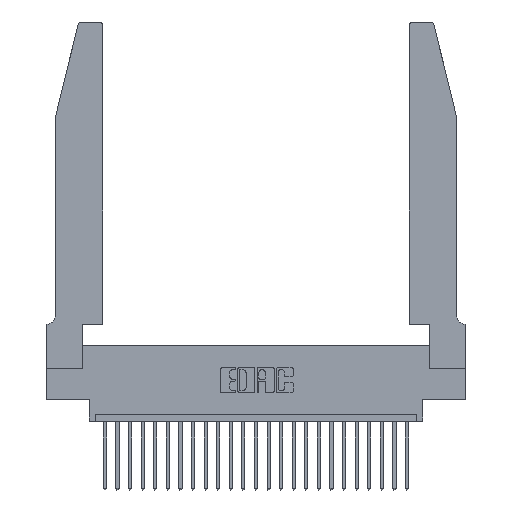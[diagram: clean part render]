
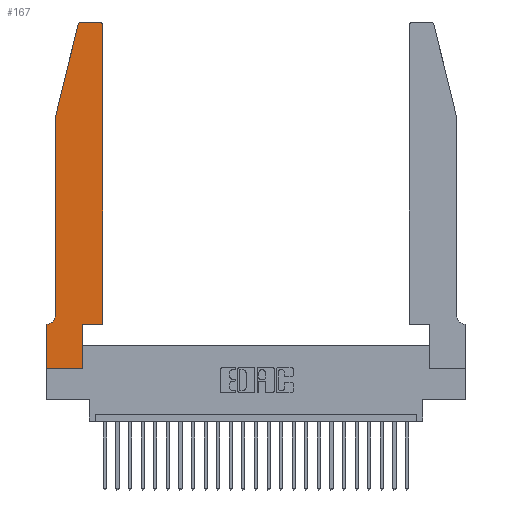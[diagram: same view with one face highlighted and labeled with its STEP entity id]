
A CAD part, top view. The second image highlights one B-rep face of the part: STEP entity #167.
In plain terms, the highlighted planar face has unit normal (0, 0, 1).
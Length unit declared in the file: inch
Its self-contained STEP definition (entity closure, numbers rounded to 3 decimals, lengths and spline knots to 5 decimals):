
#39 = DIRECTION ( 'NONE',  ( -1., 0., 0. ) ) ;
#167 = ADVANCED_FACE ( 'NONE', ( #18396 ), #13384, .T. ) ;
#365 = DIRECTION ( 'NONE',  ( 0., -1., 0. ) ) ;
#566 = VERTEX_POINT ( 'NONE', #7921 ) ;
#582 = CARTESIAN_POINT ( 'NONE',  ( 0.284, 2.72, 0.37 ) ) ;
#617 = VERTEX_POINT ( 'NONE', #24511 ) ;
#814 = EDGE_CURVE ( 'NONE', #566, #20338, #5829, .T. ) ;
#999 = VERTEX_POINT ( 'NONE', #2072 ) ;
#1170 = DIRECTION ( 'NONE',  ( 1., 0., 0. ) ) ;
#1643 = VECTOR ( 'NONE', #13195, 39.37008 ) ;
#1770 = ORIENTED_EDGE ( 'NONE', *, *, #11974, .T. ) ;
#1819 = LINE ( 'NONE', #13498, #22578 ) ;
#2072 = CARTESIAN_POINT ( 'NONE',  ( 0.4505, 0.35, 0.37 ) ) ;
#2327 = LINE ( 'NONE', #6353, #23367 ) ;
#2420 = EDGE_CURVE ( 'NONE', #9764, #12664, #5429, .T. ) ;
#2441 = LINE ( 'NONE', #2659, #17865 ) ;
#2659 = CARTESIAN_POINT ( 'NONE',  ( 0., 0., 0.37 ) ) ;
#3361 = ORIENTED_EDGE ( 'NONE', *, *, #10811, .T. ) ;
#4263 = DIRECTION ( 'NONE',  ( -1., 0., 0. ) ) ;
#4925 = EDGE_CURVE ( 'NONE', #22649, #25336, #2441, .T. ) ;
#5098 = CARTESIAN_POINT ( 'NONE',  ( 0.4505, 0.35, 0.37 ) ) ;
#5145 = LINE ( 'NONE', #5098, #1643 ) ;
#5199 = CARTESIAN_POINT ( 'NONE',  ( 0.0755, 2., 0.37 ) ) ;
#5429 = CIRCLE ( 'NONE', #22762, 0.07 ) ;
#5458 = AXIS2_PLACEMENT_3D ( 'NONE', #582, #18688, #22543 ) ;
#5829 = CIRCLE ( 'NONE', #11359, 0.03 ) ;
#5853 = LINE ( 'NONE', #8054, #14052 ) ;
#6013 = DIRECTION ( 'NONE',  ( 1., 0., 0. ) ) ;
#6155 = EDGE_LOOP ( 'NONE', ( #20588, #1770, #6347, #13376, #12126, #21054, #19779, #21338, #3361, #15868, #18955, #24180 ) ) ;
#6347 = ORIENTED_EDGE ( 'NONE', *, *, #15569, .T. ) ;
#6353 = CARTESIAN_POINT ( 'NONE',  ( 0.0755, 0.35, 0.37 ) ) ;
#6870 = EDGE_CURVE ( 'NONE', #25336, #15212, #14333, .T. ) ;
#6914 = CARTESIAN_POINT ( 'NONE',  ( 0.0055, 0.42, 0.37 ) ) ;
#7462 = DIRECTION ( 'NONE',  ( -0.239, -0.971, 0. ) ) ;
#7697 = VERTEX_POINT ( 'NONE', #20103 ) ;
#7700 = VECTOR ( 'NONE', #7462, 39.37008 ) ;
#7833 = VERTEX_POINT ( 'NONE', #9425 ) ;
#7921 = CARTESIAN_POINT ( 'NONE',  ( 0.4505, 2.72, 0.37 ) ) ;
#8054 = CARTESIAN_POINT ( 'NONE',  ( 0.2605, 2.75, 0.37 ) ) ;
#8765 = VECTOR ( 'NONE', #24803, 39.37008 ) ;
#9080 = CARTESIAN_POINT ( 'NONE',  ( 0., 0.35, 0.37 ) ) ;
#9425 = CARTESIAN_POINT ( 'NONE',  ( 0.25487, 2.72718, 0.37 ) ) ;
#9755 = CARTESIAN_POINT ( 'NONE',  ( 0.0755, 2., 0.37 ) ) ;
#9764 = VERTEX_POINT ( 'NONE', #16952 ) ;
#10227 = CARTESIAN_POINT ( 'NONE',  ( 0., 0.35, 0.37 ) ) ;
#10811 = EDGE_CURVE ( 'NONE', #15212, #617, #1819, .T. ) ;
#11359 = AXIS2_PLACEMENT_3D ( 'NONE', #23527, #21575, #11745 ) ;
#11745 = DIRECTION ( 'NONE',  ( 1., 0., 0. ) ) ;
#11974 = EDGE_CURVE ( 'NONE', #7697, #7833, #23511, .T. ) ;
#12126 = ORIENTED_EDGE ( 'NONE', *, *, #2420, .T. ) ;
#12551 = LINE ( 'NONE', #5199, #8765 ) ;
#12664 = VERTEX_POINT ( 'NONE', #19971 ) ;
#13054 = LINE ( 'NONE', #9755, #7700 ) ;
#13195 = DIRECTION ( 'NONE',  ( 0., 1., 0. ) ) ;
#13289 = DIRECTION ( 'NONE',  ( 0., 0., 1. ) ) ;
#13306 = EDGE_CURVE ( 'NONE', #18325, #9764, #12551, .T. ) ;
#13376 = ORIENTED_EDGE ( 'NONE', *, *, #13306, .T. ) ;
#13384 = PLANE ( 'NONE',  #23894 ) ;
#13498 = CARTESIAN_POINT ( 'NONE',  ( 0.2865, 0.35, 0.37 ) ) ;
#13594 = DIRECTION ( 'NONE',  ( 0., 1., 0. ) ) ;
#13707 = VECTOR ( 'NONE', #16225, 39.37008 ) ;
#14052 = VECTOR ( 'NONE', #4263, 39.37008 ) ;
#14333 = LINE ( 'NONE', #20367, #13707 ) ;
#15212 = VERTEX_POINT ( 'NONE', #15760 ) ;
#15569 = EDGE_CURVE ( 'NONE', #7833, #18325, #13054, .T. ) ;
#15760 = CARTESIAN_POINT ( 'NONE',  ( 0.2865, 0., 0.37 ) ) ;
#15868 = ORIENTED_EDGE ( 'NONE', *, *, #16824, .T. ) ;
#15955 = EDGE_CURVE ( 'NONE', #999, #566, #5145, .T. ) ;
#16225 = DIRECTION ( 'NONE',  ( 1., 0., 0. ) ) ;
#16824 = EDGE_CURVE ( 'NONE', #617, #999, #22338, .T. ) ;
#16952 = CARTESIAN_POINT ( 'NONE',  ( 0.0755, 0.42, 0.37 ) ) ;
#17274 = CARTESIAN_POINT ( 'NONE',  ( 0.4205, 2.75, 0.37 ) ) ;
#17865 = VECTOR ( 'NONE', #365, 39.37008 ) ;
#17932 = CARTESIAN_POINT ( 'NONE',  ( 0., 0., 0.37 ) ) ;
#18017 = CARTESIAN_POINT ( 'NONE',  ( 0.4505, 0.35, 0.37 ) ) ;
#18325 = VERTEX_POINT ( 'NONE', #20855 ) ;
#18396 = FACE_OUTER_BOUND ( 'NONE', #6155, .T. ) ;
#18688 = DIRECTION ( 'NONE',  ( 0., 0., 1. ) ) ;
#18955 = ORIENTED_EDGE ( 'NONE', *, *, #15955, .T. ) ;
#19207 = VECTOR ( 'NONE', #6013, 39.37008 ) ;
#19779 = ORIENTED_EDGE ( 'NONE', *, *, #4925, .T. ) ;
#19971 = CARTESIAN_POINT ( 'NONE',  ( 0.0055, 0.35, 0.37 ) ) ;
#20103 = CARTESIAN_POINT ( 'NONE',  ( 0.284, 2.75, 0.37 ) ) ;
#20338 = VERTEX_POINT ( 'NONE', #17274 ) ;
#20367 = CARTESIAN_POINT ( 'NONE',  ( 0., 0., 0.37 ) ) ;
#20588 = ORIENTED_EDGE ( 'NONE', *, *, #23816, .T. ) ;
#20855 = CARTESIAN_POINT ( 'NONE',  ( 0.0755, 2., 0.37 ) ) ;
#20964 = DIRECTION ( 'NONE',  ( -1., 0., 0. ) ) ;
#21054 = ORIENTED_EDGE ( 'NONE', *, *, #24378, .T. ) ;
#21338 = ORIENTED_EDGE ( 'NONE', *, *, #6870, .T. ) ;
#21575 = DIRECTION ( 'NONE',  ( 0., 0., 1. ) ) ;
#22338 = LINE ( 'NONE', #18017, #19207 ) ;
#22543 = DIRECTION ( 'NONE',  ( 1., 0., 0. ) ) ;
#22578 = VECTOR ( 'NONE', #13594, 39.37008 ) ;
#22649 = VERTEX_POINT ( 'NONE', #10227 ) ;
#22762 = AXIS2_PLACEMENT_3D ( 'NONE', #6914, #23171, #20964 ) ;
#23171 = DIRECTION ( 'NONE',  ( 0., 0., -1. ) ) ;
#23367 = VECTOR ( 'NONE', #39, 39.37008 ) ;
#23511 = CIRCLE ( 'NONE', #5458, 0.03 ) ;
#23527 = CARTESIAN_POINT ( 'NONE',  ( 0.4205, 2.72, 0.37 ) ) ;
#23816 = EDGE_CURVE ( 'NONE', #20338, #7697, #5853, .T. ) ;
#23894 = AXIS2_PLACEMENT_3D ( 'NONE', #9080, #13289, #1170 ) ;
#24180 = ORIENTED_EDGE ( 'NONE', *, *, #814, .T. ) ;
#24378 = EDGE_CURVE ( 'NONE', #12664, #22649, #2327, .T. ) ;
#24511 = CARTESIAN_POINT ( 'NONE',  ( 0.2865, 0.35, 0.37 ) ) ;
#24803 = DIRECTION ( 'NONE',  ( 0., -1., 0. ) ) ;
#25336 = VERTEX_POINT ( 'NONE', #17932 ) ;
